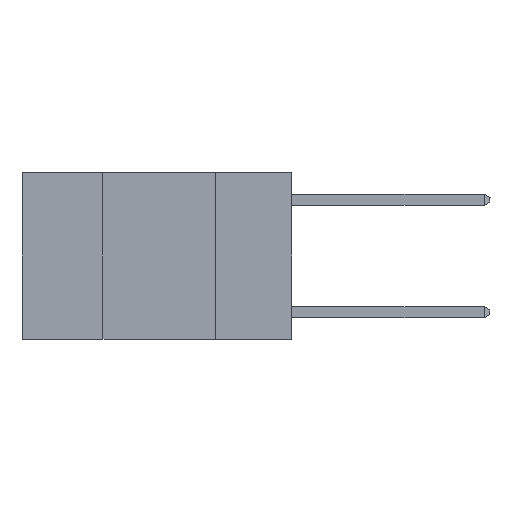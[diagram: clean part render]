
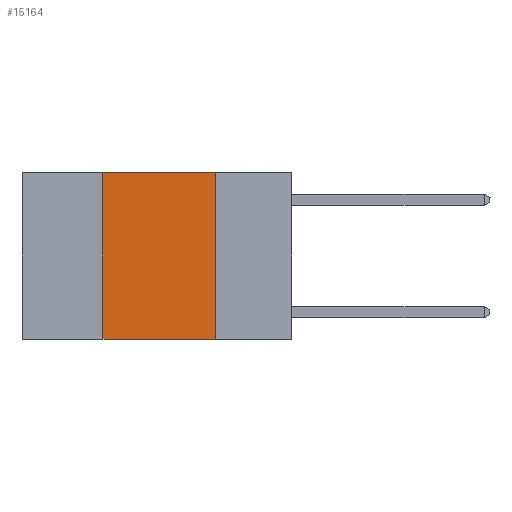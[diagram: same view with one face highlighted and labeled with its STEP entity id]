
A CAD part, left-side view. The second image highlights one B-rep face of the part: STEP entity #15164.
In plain terms, the highlighted planar face has unit normal (-1, 0, 0).
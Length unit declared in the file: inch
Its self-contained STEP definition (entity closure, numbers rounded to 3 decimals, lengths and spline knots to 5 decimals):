
#11 = DIRECTION ( 'NONE',  ( 0., -1., 0. ) ) ;
#112 = LINE ( 'NONE', #13415, #2742 ) ;
#485 = CARTESIAN_POINT ( 'NONE',  ( 0., 0.42, -0.37 ) ) ;
#766 = DIRECTION ( 'NONE',  ( 1., 0., 0. ) ) ;
#934 = ORIENTED_EDGE ( 'NONE', *, *, #12220, .F. ) ;
#2472 = CARTESIAN_POINT ( 'NONE',  ( 0., 0.17, 0. ) ) ;
#2742 = VECTOR ( 'NONE', #20052, 39.37008 ) ;
#3608 = AXIS2_PLACEMENT_3D ( 'NONE', #5442, #766, #11995 ) ;
#4025 = FACE_OUTER_BOUND ( 'NONE', #7759, .T. ) ;
#4138 = EDGE_CURVE ( 'NONE', #5312, #11613, #5001, .T. ) ;
#4830 = CARTESIAN_POINT ( 'NONE',  ( 0., 0.6, -0.37 ) ) ;
#5001 = LINE ( 'NONE', #16759, #19363 ) ;
#5312 = VERTEX_POINT ( 'NONE', #11054 ) ;
#5442 = CARTESIAN_POINT ( 'NONE',  ( 0., 0.6, 0. ) ) ;
#5457 = EDGE_CURVE ( 'NONE', #8211, #5312, #112, .T. ) ;
#7308 = PLANE ( 'NONE',  #3608 ) ;
#7466 = VERTEX_POINT ( 'NONE', #16839 ) ;
#7759 = EDGE_LOOP ( 'NONE', ( #934, #17973, #20097, #13833 ) ) ;
#8211 = VERTEX_POINT ( 'NONE', #485 ) ;
#8654 = LINE ( 'NONE', #4830, #18515 ) ;
#11021 = EDGE_CURVE ( 'NONE', #8211, #7466, #8654, .T. ) ;
#11054 = CARTESIAN_POINT ( 'NONE',  ( 0., 0.42, 0. ) ) ;
#11613 = VERTEX_POINT ( 'NONE', #18750 ) ;
#11995 = DIRECTION ( 'NONE',  ( 0., 0., -1. ) ) ;
#12220 = EDGE_CURVE ( 'NONE', #11613, #7466, #14154, .T. ) ;
#13415 = CARTESIAN_POINT ( 'NONE',  ( 0., 0.42, 0. ) ) ;
#13833 = ORIENTED_EDGE ( 'NONE', *, *, #11021, .T. ) ;
#14154 = LINE ( 'NONE', #2472, #21357 ) ;
#15164 = ADVANCED_FACE ( 'NONE', ( #4025 ), #7308, .F. ) ;
#15879 = DIRECTION ( 'NONE',  ( 0., 0., -1. ) ) ;
#16759 = CARTESIAN_POINT ( 'NONE',  ( 0., 0.6, 0. ) ) ;
#16839 = CARTESIAN_POINT ( 'NONE',  ( 0., 0.17, -0.37 ) ) ;
#17973 = ORIENTED_EDGE ( 'NONE', *, *, #4138, .F. ) ;
#18338 = DIRECTION ( 'NONE',  ( 0., -1., 0. ) ) ;
#18515 = VECTOR ( 'NONE', #18338, 39.37008 ) ;
#18750 = CARTESIAN_POINT ( 'NONE',  ( 0., 0.17, 0. ) ) ;
#19363 = VECTOR ( 'NONE', #11, 39.37008 ) ;
#20052 = DIRECTION ( 'NONE',  ( 0., 0., 1. ) ) ;
#20097 = ORIENTED_EDGE ( 'NONE', *, *, #5457, .F. ) ;
#21357 = VECTOR ( 'NONE', #15879, 39.37008 ) ;
